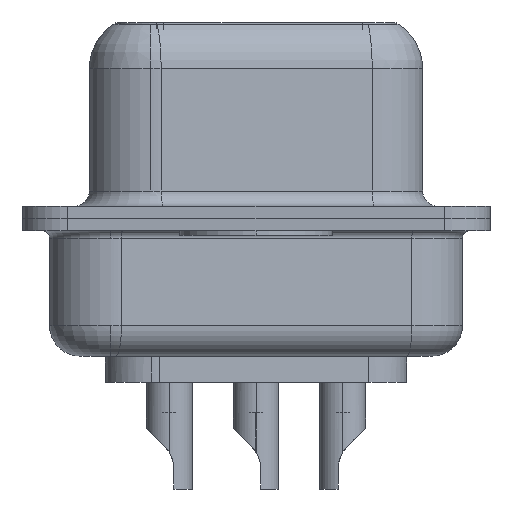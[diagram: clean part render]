
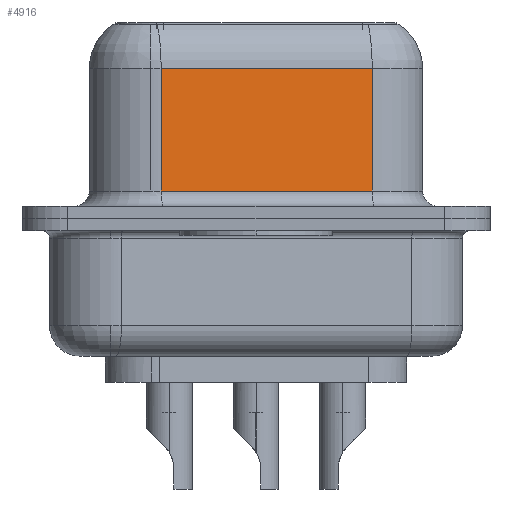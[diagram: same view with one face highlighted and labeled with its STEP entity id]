
A CAD part, left-side view. The second image highlights one B-rep face of the part: STEP entity #4916.
In plain terms, the highlighted planar face has unit normal (-0.985, -0.174, 0).
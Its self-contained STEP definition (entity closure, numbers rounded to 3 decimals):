
#481 = LINE ( 'NONE', #7776, #670 ) ;
#670 = VECTOR ( 'NONE', #17458, 1000. ) ;
#1052 = VECTOR ( 'NONE', #4672, 1000. ) ;
#2215 = EDGE_CURVE ( 'NONE', #11558, #17638, #18910, .T. ) ;
#3982 = DIRECTION ( 'NONE',  ( 0., 0., -1. ) ) ;
#4038 = FACE_OUTER_BOUND ( 'NONE', #28564, .T. ) ;
#4478 = CARTESIAN_POINT ( 'NONE',  ( 5.647, -3.797, 0.9 ) ) ;
#4672 = DIRECTION ( 'NONE',  ( 0.174, -0.985, 0. ) ) ;
#4916 = ADVANCED_FACE ( 'NONE', ( #4038 ), #18636, .F. ) ;
#4969 = LINE ( 'NONE', #14176, #1052 ) ;
#5477 = EDGE_CURVE ( 'NONE', #22635, #11558, #481, .T. ) ;
#6568 = DIRECTION ( 'NONE',  ( 0.985, 0.174, 0. ) ) ;
#7776 = CARTESIAN_POINT ( 'NONE',  ( 5.647, -3.797, 4.9 ) ) ;
#8428 = CARTESIAN_POINT ( 'NONE',  ( 4.43, 3.103, 0.9 ) ) ;
#9640 = ORIENTED_EDGE ( 'NONE', *, *, #13198, .T. ) ;
#10863 = VECTOR ( 'NONE', #3982, 1000. ) ;
#11558 = VERTEX_POINT ( 'NONE', #16902 ) ;
#13198 = EDGE_CURVE ( 'NONE', #17638, #23041, #4969, .T. ) ;
#14176 = CARTESIAN_POINT ( 'NONE',  ( 5.647, -3.797, 0.9 ) ) ;
#14392 = ORIENTED_EDGE ( 'NONE', *, *, #2215, .T. ) ;
#14438 = DIRECTION ( 'NONE',  ( 0., 0., -1. ) ) ;
#14854 = ORIENTED_EDGE ( 'NONE', *, *, #27580, .F. ) ;
#16902 = CARTESIAN_POINT ( 'NONE',  ( 4.43, 3.103, 4.9 ) ) ;
#17458 = DIRECTION ( 'NONE',  ( -0.174, 0.985, 0. ) ) ;
#17638 = VERTEX_POINT ( 'NONE', #8428 ) ;
#18266 = CARTESIAN_POINT ( 'NONE',  ( 5.647, -3.797, 6.65 ) ) ;
#18333 = AXIS2_PLACEMENT_3D ( 'NONE', #28327, #6568, #21977 ) ;
#18636 = PLANE ( 'NONE',  #18333 ) ;
#18910 = LINE ( 'NONE', #21618, #27803 ) ;
#21618 = CARTESIAN_POINT ( 'NONE',  ( 4.43, 3.103, 6.65 ) ) ;
#21977 = DIRECTION ( 'NONE',  ( -0.174, 0.985, 0. ) ) ;
#22635 = VERTEX_POINT ( 'NONE', #26590 ) ;
#23041 = VERTEX_POINT ( 'NONE', #4478 ) ;
#26590 = CARTESIAN_POINT ( 'NONE',  ( 5.647, -3.797, 4.9 ) ) ;
#27580 = EDGE_CURVE ( 'NONE', #22635, #23041, #28269, .T. ) ;
#27803 = VECTOR ( 'NONE', #14438, 1000. ) ;
#28269 = LINE ( 'NONE', #18266, #10863 ) ;
#28327 = CARTESIAN_POINT ( 'NONE',  ( 5.647, -3.797, 6.65 ) ) ;
#28564 = EDGE_LOOP ( 'NONE', ( #14854, #29788, #14392, #9640 ) ) ;
#29788 = ORIENTED_EDGE ( 'NONE', *, *, #5477, .T. ) ;
